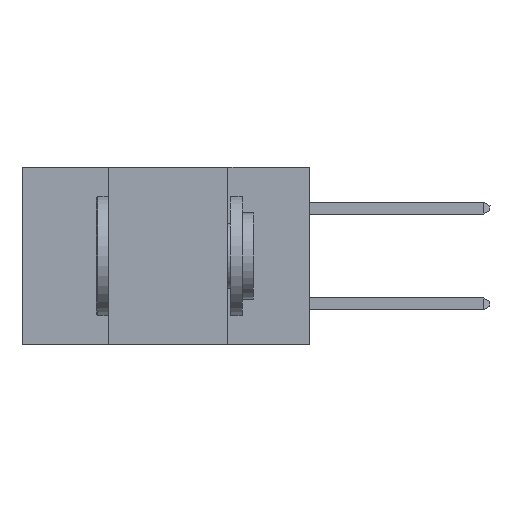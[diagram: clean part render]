
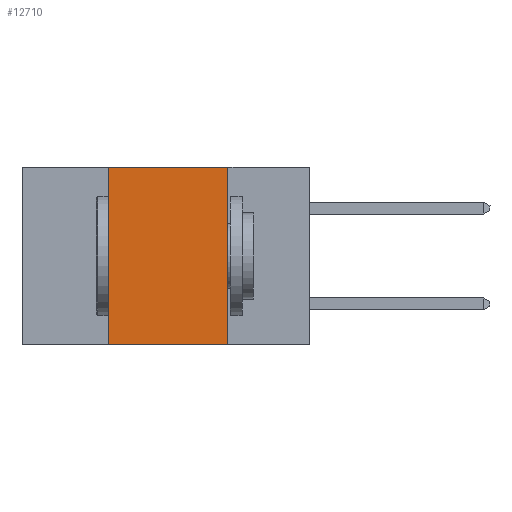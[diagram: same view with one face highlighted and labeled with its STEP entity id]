
A CAD part, left-side view. The second image highlights one B-rep face of the part: STEP entity #12710.
In plain terms, the highlighted planar face has unit normal (-1, 0, 0).
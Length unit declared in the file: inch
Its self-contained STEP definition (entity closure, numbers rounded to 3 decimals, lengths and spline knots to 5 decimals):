
#1190 = VERTEX_POINT ( 'NONE', #3661 ) ;
#3388 = CARTESIAN_POINT ( 'NONE',  ( 0., 0.42, 0. ) ) ;
#3661 = CARTESIAN_POINT ( 'NONE',  ( 0., 0.17, -0.37 ) ) ;
#4265 = CARTESIAN_POINT ( 'NONE',  ( 0., 0.42, -0.37 ) ) ;
#4484 = CARTESIAN_POINT ( 'NONE',  ( 0., 0.6, 0. ) ) ;
#4519 = VECTOR ( 'NONE', #14811, 39.37008 ) ;
#4624 = EDGE_CURVE ( 'NONE', #15655, #22048, #13713, .T. ) ;
#5390 = CARTESIAN_POINT ( 'NONE',  ( 0., 0.17, 0. ) ) ;
#5654 = EDGE_CURVE ( 'NONE', #22048, #1190, #5796, .T. ) ;
#5796 = LINE ( 'NONE', #5390, #10404 ) ;
#6071 = ORIENTED_EDGE ( 'NONE', *, *, #4624, .F. ) ;
#6577 = PLANE ( 'NONE',  #18260 ) ;
#7922 = ORIENTED_EDGE ( 'NONE', *, *, #10881, .F. ) ;
#8302 = ORIENTED_EDGE ( 'NONE', *, *, #5654, .F. ) ;
#8614 = DIRECTION ( 'NONE',  ( 0., 0., 1. ) ) ;
#8857 = DIRECTION ( 'NONE',  ( 0., 0., -1. ) ) ;
#10074 = DIRECTION ( 'NONE',  ( 1., 0., 0. ) ) ;
#10404 = VECTOR ( 'NONE', #8857, 39.37008 ) ;
#10881 = EDGE_CURVE ( 'NONE', #21145, #15655, #12886, .T. ) ;
#11789 = CARTESIAN_POINT ( 'NONE',  ( 0., 0.6, 0. ) ) ;
#12480 = EDGE_CURVE ( 'NONE', #21145, #1190, #12850, .T. ) ;
#12710 = ADVANCED_FACE ( 'NONE', ( #17078 ), #6577, .F. ) ;
#12850 = LINE ( 'NONE', #16334, #19501 ) ;
#12886 = LINE ( 'NONE', #3388, #16873 ) ;
#13619 = CARTESIAN_POINT ( 'NONE',  ( 0., 0.42, 0. ) ) ;
#13713 = LINE ( 'NONE', #4484, #4519 ) ;
#14811 = DIRECTION ( 'NONE',  ( 0., -1., 0. ) ) ;
#15274 = EDGE_LOOP ( 'NONE', ( #8302, #6071, #7922, #17030 ) ) ;
#15655 = VERTEX_POINT ( 'NONE', #13619 ) ;
#16334 = CARTESIAN_POINT ( 'NONE',  ( 0., 0.6, -0.37 ) ) ;
#16873 = VECTOR ( 'NONE', #8614, 39.37008 ) ;
#17030 = ORIENTED_EDGE ( 'NONE', *, *, #12480, .T. ) ;
#17078 = FACE_OUTER_BOUND ( 'NONE', #15274, .T. ) ;
#18260 = AXIS2_PLACEMENT_3D ( 'NONE', #11789, #10074, #21989 ) ;
#19501 = VECTOR ( 'NONE', #19779, 39.37008 ) ;
#19779 = DIRECTION ( 'NONE',  ( 0., -1., 0. ) ) ;
#20408 = CARTESIAN_POINT ( 'NONE',  ( 0., 0.17, 0. ) ) ;
#21145 = VERTEX_POINT ( 'NONE', #4265 ) ;
#21989 = DIRECTION ( 'NONE',  ( 0., 0., -1. ) ) ;
#22048 = VERTEX_POINT ( 'NONE', #20408 ) ;
